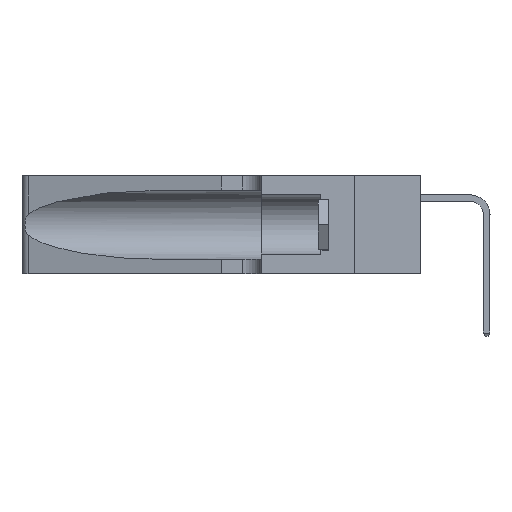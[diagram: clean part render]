
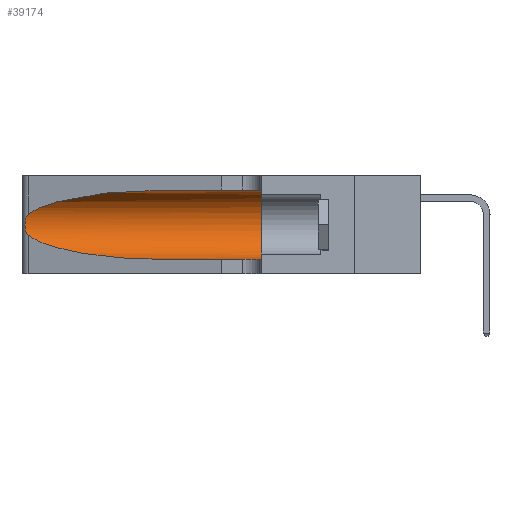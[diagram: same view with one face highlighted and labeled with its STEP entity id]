
A CAD part, left-side view. The second image highlights one B-rep face of the part: STEP entity #39174.
In plain terms, the highlighted cylindrical face has radius 3.308 mm (diameter 6.617 mm), a partial arc.
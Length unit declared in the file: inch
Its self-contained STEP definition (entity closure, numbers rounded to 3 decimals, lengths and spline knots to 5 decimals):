
#1971 = CARTESIAN_POINT ( 'NONE',  ( 0.1305, 0.72297, 0.05475 ) ) ;
#2192 = ORIENTED_EDGE ( 'NONE', *, *, #5529, .T. ) ;
#2521 = CARTESIAN_POINT ( 'NONE',  ( 0.25555, 1.22993, 0.14849 ) ) ;
#5518 = CARTESIAN_POINT ( 'NONE',  ( 0.18966, 0.96281, 0.05475 ) ) ;
#5529 = EDGE_CURVE ( 'NONE', #46325, #33552, #15283, .T. ) ;
#6757 = ORIENTED_EDGE ( 'NONE', *, *, #29703, .T. ) ;
#7120 = FACE_OUTER_BOUND ( 'NONE', #18149, .T. ) ;
#7190 = CARTESIAN_POINT ( 'NONE',  ( 0.1305, 0.35, 0.05475 ) ) ;
#9058 = CARTESIAN_POINT ( 'NONE',  ( 0.2373, 1.15595, 0.28018 ) ) ;
#9528 = CARTESIAN_POINT ( 'NONE',  ( 0.25487, 1.22718, 0.14631 ) ) ;
#9757 = CARTESIAN_POINT ( 'NONE',  ( 0.25787, 1.23484, 0.2124 ) ) ;
#11305 = DIRECTION ( 'NONE',  ( 0., 1., 0. ) ) ;
#11799 = CARTESIAN_POINT ( 'NONE',  ( 0.1305, 1.61858, 0.31525 ) ) ;
#12960 = VERTEX_POINT ( 'NONE', #16556 ) ;
#13414 = CARTESIAN_POINT ( 'NONE',  ( 0.26018, 1.23835, 0.19895 ) ) ;
#13840 = DIRECTION ( 'NONE',  ( 0., -1., 0. ) ) ;
#14770 = ORIENTED_EDGE ( 'NONE', *, *, #38049, .T. ) ;
#15283 = LINE ( 'NONE', #24474, #42862 ) ;
#15477 = CARTESIAN_POINT ( 'NONE',  ( 0.1305, 1.61858, 0.185 ) ) ;
#15663 = CYLINDRICAL_SURFACE ( 'NONE', #38107, 0.13025 ) ;
#16101 = LINE ( 'NONE', #11799, #17226 ) ;
#16556 = CARTESIAN_POINT ( 'NONE',  ( 0.1305, 0.72297, 0.31525 ) ) ;
#17029 = CARTESIAN_POINT ( 'NONE',  ( 0.26075, 1.23896, 0.178 ) ) ;
#17109 =( BOUNDED_CURVE ( )  B_SPLINE_CURVE ( 3, ( #23517, #45136, #5518, #30740 ),
 .UNSPECIFIED., .F., .F. ) 
 B_SPLINE_CURVE_WITH_KNOTS ( ( 4, 4 ),
 ( 3.44316, 4.71239 ),
 .UNSPECIFIED. ) 
 CURVE ( )  GEOMETRIC_REPRESENTATION_ITEM ( )  RATIONAL_B_SPLINE_CURVE ( ( 1., 0.87, 0.87, 1. ) ) 
 REPRESENTATION_ITEM ( '' )  );
#17226 = VECTOR ( 'NONE', #29817, 39.37008 ) ;
#17988 = EDGE_CURVE ( 'NONE', #12960, #26739, #20940, .T. ) ;
#18108 = ORIENTED_EDGE ( 'NONE', *, *, #17988, .T. ) ;
#18149 = EDGE_LOOP ( 'NONE', ( #18108, #6757, #14770, #2192, #33863, #20025 ) ) ;
#18382 = B_SPLINE_CURVE_WITH_KNOTS ( 'NONE', 3,
 ( #20446, #45663, #31272, #9757, #34909, #13414, #38563, #17029, #42196, #20588, #45827, #24200, #2521, #27815 ),
 .UNSPECIFIED., .F., .F.,
 ( 4, 2, 2, 2, 2, 2, 4 ),
 ( 0., 0.00027, 0.00053, 0.00107, 0.0016, 0.00187, 0.00214 ),
 .UNSPECIFIED. ) ;
#20025 = ORIENTED_EDGE ( 'NONE', *, *, #37865, .F. ) ;
#20446 = CARTESIAN_POINT ( 'NONE',  ( 0.25487, 1.22718, 0.22369 ) ) ;
#20588 = CARTESIAN_POINT ( 'NONE',  ( 0.25856, 1.23593, 0.16098 ) ) ;
#20940 =( BOUNDED_CURVE ( )  B_SPLINE_CURVE ( 3, ( #23369, #26982, #9058, #34216 ),
 .UNSPECIFIED., .F., .T. ) 
 B_SPLINE_CURVE_WITH_KNOTS ( ( 4, 4 ),
 ( 1.5708, 2.84003 ),
 .UNSPECIFIED. ) 
 CURVE ( )  GEOMETRIC_REPRESENTATION_ITEM ( )  RATIONAL_B_SPLINE_CURVE ( ( 1., 0.87, 0.87, 1. ) ) 
 REPRESENTATION_ITEM ( '' )  );
#21408 = CIRCLE ( 'NONE', #27217, 0.13025 ) ;
#23369 = CARTESIAN_POINT ( 'NONE',  ( 0.1305, 0.72297, 0.31525 ) ) ;
#23517 = CARTESIAN_POINT ( 'NONE',  ( 0.25487, 1.22718, 0.14631 ) ) ;
#24200 = CARTESIAN_POINT ( 'NONE',  ( 0.25639, 1.23186, 0.15144 ) ) ;
#24474 = CARTESIAN_POINT ( 'NONE',  ( 0.1305, 1.61858, 0.05475 ) ) ;
#26256 = DIRECTION ( 'NONE',  ( 0., -1., 0. ) ) ;
#26739 = VERTEX_POINT ( 'NONE', #27042 ) ;
#26982 = CARTESIAN_POINT ( 'NONE',  ( 0.18966, 0.96281, 0.31525 ) ) ;
#27042 = CARTESIAN_POINT ( 'NONE',  ( 0.25487, 1.22718, 0.22369 ) ) ;
#27217 = AXIS2_PLACEMENT_3D ( 'NONE', #32801, #11305, #36420 ) ;
#27815 = CARTESIAN_POINT ( 'NONE',  ( 0.25487, 1.22718, 0.14631 ) ) ;
#28570 = VERTEX_POINT ( 'NONE', #35948 ) ;
#29703 = EDGE_CURVE ( 'NONE', #26739, #38096, #18382, .T. ) ;
#29817 = DIRECTION ( 'NONE',  ( 0., -1., 0. ) ) ;
#30740 = CARTESIAN_POINT ( 'NONE',  ( 0.1305, 0.72297, 0.05475 ) ) ;
#31272 = CARTESIAN_POINT ( 'NONE',  ( 0.25639, 1.23184, 0.21858 ) ) ;
#32801 = CARTESIAN_POINT ( 'NONE',  ( 0.1305, 0.35, 0.185 ) ) ;
#33482 = DIRECTION ( 'NONE',  ( 0., 0., -1. ) ) ;
#33552 = VERTEX_POINT ( 'NONE', #7190 ) ;
#33863 = ORIENTED_EDGE ( 'NONE', *, *, #34303, .F. ) ;
#34216 = CARTESIAN_POINT ( 'NONE',  ( 0.25487, 1.22718, 0.22369 ) ) ;
#34303 = EDGE_CURVE ( 'NONE', #28570, #33552, #21408, .T. ) ;
#34909 = CARTESIAN_POINT ( 'NONE',  ( 0.25854, 1.2359, 0.20912 ) ) ;
#35948 = CARTESIAN_POINT ( 'NONE',  ( 0.1305, 0.35, 0.31525 ) ) ;
#36420 = DIRECTION ( 'NONE',  ( 0., 0., 1. ) ) ;
#37865 = EDGE_CURVE ( 'NONE', #12960, #28570, #16101, .T. ) ;
#38049 = EDGE_CURVE ( 'NONE', #38096, #46325, #17109, .T. ) ;
#38096 = VERTEX_POINT ( 'NONE', #9528 ) ;
#38107 = AXIS2_PLACEMENT_3D ( 'NONE', #15477, #26256, #33482 ) ;
#38563 = CARTESIAN_POINT ( 'NONE',  ( 0.26075, 1.23896, 0.19203 ) ) ;
#39174 = ADVANCED_FACE ( 'NONE', ( #7120 ), #15663, .F. ) ;
#42196 = CARTESIAN_POINT ( 'NONE',  ( 0.26017, 1.23833, 0.17102 ) ) ;
#42862 = VECTOR ( 'NONE', #13840, 39.37008 ) ;
#45136 = CARTESIAN_POINT ( 'NONE',  ( 0.2373, 1.15595, 0.08982 ) ) ;
#45663 = CARTESIAN_POINT ( 'NONE',  ( 0.25555, 1.22994, 0.2215 ) ) ;
#45827 = CARTESIAN_POINT ( 'NONE',  ( 0.25789, 1.23486, 0.15765 ) ) ;
#46325 = VERTEX_POINT ( 'NONE', #1971 ) ;
